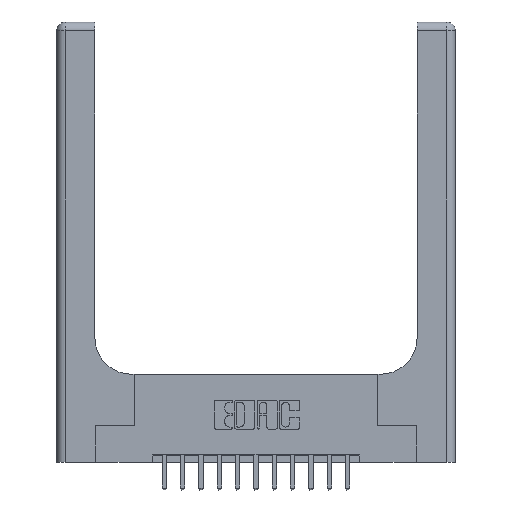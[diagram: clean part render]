
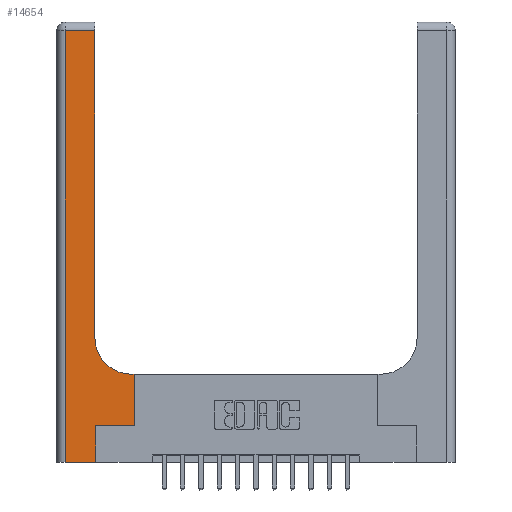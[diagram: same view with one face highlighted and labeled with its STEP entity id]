
A CAD part, top view. The second image highlights one B-rep face of the part: STEP entity #14654.
In plain terms, the highlighted planar face has unit normal (0, 0, 1).
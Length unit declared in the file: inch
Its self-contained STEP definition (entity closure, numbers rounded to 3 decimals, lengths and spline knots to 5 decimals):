
#81 = EDGE_CURVE ( 'NONE', #5696, #800, #15668, .T. ) ;
#219 = VERTEX_POINT ( 'NONE', #2194 ) ;
#433 = CARTESIAN_POINT ( 'NONE',  ( 0.26, 3., 0.37 ) ) ;
#551 = DIRECTION ( 'NONE',  ( 0., 1., 0. ) ) ;
#728 = DIRECTION ( 'NONE',  ( 1., 0., 0. ) ) ;
#800 = VERTEX_POINT ( 'NONE', #10604 ) ;
#826 = DIRECTION ( 'NONE',  ( 0., 1., 0. ) ) ;
#862 = LINE ( 'NONE', #5762, #14134 ) ;
#1003 = LINE ( 'NONE', #13284, #13872 ) ;
#1490 = AXIS2_PLACEMENT_3D ( 'NONE', #9806, #16238, #9921 ) ;
#1769 = ORIENTED_EDGE ( 'NONE', *, *, #81, .T. ) ;
#1917 = LINE ( 'NONE', #7087, #14556 ) ;
#2194 = CARTESIAN_POINT ( 'NONE',  ( 0.528, 0.25, 0.37 ) ) ;
#2441 = DIRECTION ( 'NONE',  ( 1., 0., 0. ) ) ;
#2804 = EDGE_CURVE ( 'NONE', #9228, #6131, #1917, .T. ) ;
#2856 = AXIS2_PLACEMENT_3D ( 'NONE', #13833, #6128, #2441 ) ;
#3866 = LINE ( 'NONE', #15785, #6448 ) ;
#4267 = ORIENTED_EDGE ( 'NONE', *, *, #11616, .T. ) ;
#5449 = DIRECTION ( 'NONE',  ( 1., 0., 0. ) ) ;
#5696 = VERTEX_POINT ( 'NONE', #5818 ) ;
#5762 = CARTESIAN_POINT ( 'NONE',  ( 0.06, 3., 0.37 ) ) ;
#5818 = CARTESIAN_POINT ( 'NONE',  ( 0.26, 0.85, 0.37 ) ) ;
#5876 = LINE ( 'NONE', #16220, #15718 ) ;
#6128 = DIRECTION ( 'NONE',  ( 0., 0., -1. ) ) ;
#6131 = VERTEX_POINT ( 'NONE', #15749 ) ;
#6340 = VERTEX_POINT ( 'NONE', #7202 ) ;
#6448 = VECTOR ( 'NONE', #5449, 39.37008 ) ;
#7087 = CARTESIAN_POINT ( 'NONE',  ( 0., 0., 0.37 ) ) ;
#7143 = ORIENTED_EDGE ( 'NONE', *, *, #9290, .T. ) ;
#7199 = PLANE ( 'NONE',  #1490 ) ;
#7202 = CARTESIAN_POINT ( 'NONE',  ( 0.06, 2.94, 0.37 ) ) ;
#7440 = ORIENTED_EDGE ( 'NONE', *, *, #11982, .T. ) ;
#7946 = ORIENTED_EDGE ( 'NONE', *, *, #2804, .T. ) ;
#8079 = EDGE_CURVE ( 'NONE', #11549, #219, #3866, .T. ) ;
#8492 = ORIENTED_EDGE ( 'NONE', *, *, #10942, .T. ) ;
#8993 = EDGE_CURVE ( 'NONE', #9483, #10217, #1003, .T. ) ;
#9228 = VERTEX_POINT ( 'NONE', #11490 ) ;
#9273 = CARTESIAN_POINT ( 'NONE',  ( 0.528, 0.6, 0.37 ) ) ;
#9290 = EDGE_CURVE ( 'NONE', #10217, #5696, #13032, .T. ) ;
#9483 = VERTEX_POINT ( 'NONE', #9273 ) ;
#9619 = DIRECTION ( 'NONE',  ( 0., -1., 0. ) ) ;
#9806 = CARTESIAN_POINT ( 'NONE',  ( 0., 3., 0.37 ) ) ;
#9921 = DIRECTION ( 'NONE',  ( -1., 0., 0. ) ) ;
#10217 = VERTEX_POINT ( 'NONE', #13681 ) ;
#10445 = ORIENTED_EDGE ( 'NONE', *, *, #11309, .T. ) ;
#10481 = VECTOR ( 'NONE', #13131, 39.37008 ) ;
#10601 = VECTOR ( 'NONE', #551, 39.37008 ) ;
#10604 = CARTESIAN_POINT ( 'NONE',  ( 0.26, 2.94, 0.37 ) ) ;
#10942 = EDGE_CURVE ( 'NONE', #6131, #11549, #16396, .T. ) ;
#11213 = ORIENTED_EDGE ( 'NONE', *, *, #8079, .T. ) ;
#11309 = EDGE_CURVE ( 'NONE', #800, #6340, #13957, .T. ) ;
#11404 = CARTESIAN_POINT ( 'NONE',  ( 0.265, 0., 0.37 ) ) ;
#11490 = CARTESIAN_POINT ( 'NONE',  ( 0.06, 0., 0.37 ) ) ;
#11549 = VERTEX_POINT ( 'NONE', #12304 ) ;
#11616 = EDGE_CURVE ( 'NONE', #219, #9483, #5876, .T. ) ;
#11982 = EDGE_CURVE ( 'NONE', #6340, #9228, #862, .T. ) ;
#11988 = ORIENTED_EDGE ( 'NONE', *, *, #8993, .T. ) ;
#12304 = CARTESIAN_POINT ( 'NONE',  ( 0.265, 0.25, 0.37 ) ) ;
#12570 = EDGE_LOOP ( 'NONE', ( #1769, #10445, #7440, #7946, #8492, #11213, #4267, #11988, #7143 ) ) ;
#12824 = FACE_OUTER_BOUND ( 'NONE', #12570, .T. ) ;
#13032 = CIRCLE ( 'NONE', #2856, 0.25 ) ;
#13131 = DIRECTION ( 'NONE',  ( -1., 0., 0. ) ) ;
#13284 = CARTESIAN_POINT ( 'NONE',  ( 0.26, 0.6, 0.37 ) ) ;
#13681 = CARTESIAN_POINT ( 'NONE',  ( 0.51, 0.6, 0.37 ) ) ;
#13833 = CARTESIAN_POINT ( 'NONE',  ( 0.51, 0.85, 0.37 ) ) ;
#13872 = VECTOR ( 'NONE', #15414, 39.37008 ) ;
#13942 = DIRECTION ( 'NONE',  ( 0., 1., 0. ) ) ;
#13957 = LINE ( 'NONE', #14533, #10481 ) ;
#14134 = VECTOR ( 'NONE', #9619, 39.37008 ) ;
#14533 = CARTESIAN_POINT ( 'NONE',  ( 0., 2.94, 0.37 ) ) ;
#14556 = VECTOR ( 'NONE', #728, 39.37008 ) ;
#14654 = ADVANCED_FACE ( 'NONE', ( #12824 ), #7199, .F. ) ;
#15188 = VECTOR ( 'NONE', #13942, 39.37008 ) ;
#15414 = DIRECTION ( 'NONE',  ( -1., 0., 0. ) ) ;
#15668 = LINE ( 'NONE', #433, #10601 ) ;
#15718 = VECTOR ( 'NONE', #826, 39.37008 ) ;
#15749 = CARTESIAN_POINT ( 'NONE',  ( 0.265, 0., 0.37 ) ) ;
#15785 = CARTESIAN_POINT ( 'NONE',  ( 0.265, 0.25, 0.37 ) ) ;
#16220 = CARTESIAN_POINT ( 'NONE',  ( 0.528, 0.25, 0.37 ) ) ;
#16238 = DIRECTION ( 'NONE',  ( 0., 0., -1. ) ) ;
#16396 = LINE ( 'NONE', #11404, #15188 ) ;
